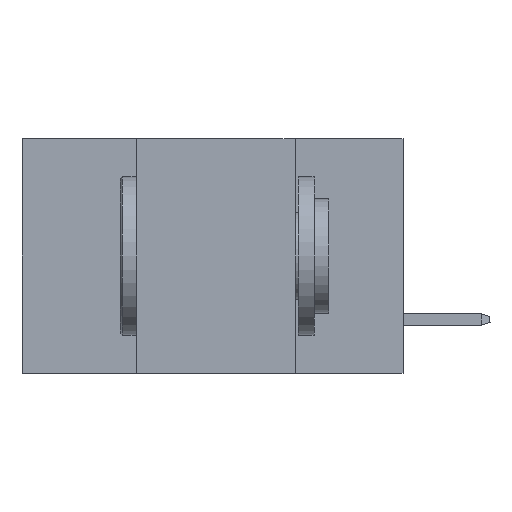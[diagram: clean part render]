
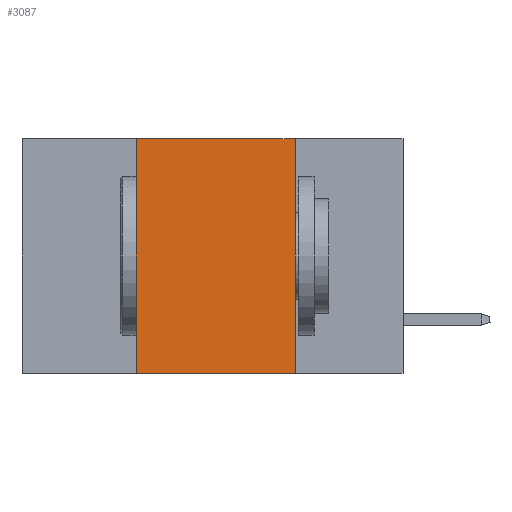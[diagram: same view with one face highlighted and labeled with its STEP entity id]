
A CAD part, left-side view. The second image highlights one B-rep face of the part: STEP entity #3087.
In plain terms, the highlighted planar face has unit normal (-1, 0, 0).
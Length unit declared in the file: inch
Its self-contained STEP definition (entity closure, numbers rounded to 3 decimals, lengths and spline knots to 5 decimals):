
#772 = LINE ( 'NONE', #17700, #2899 ) ;
#1474 = CARTESIAN_POINT ( 'NONE',  ( 0., 0.6, 0. ) ) ;
#1555 = EDGE_CURVE ( 'NONE', #10267, #7672, #14906, .T. ) ;
#1902 = VECTOR ( 'NONE', #2129, 39.37008 ) ;
#2129 = DIRECTION ( 'NONE',  ( 0., -1., 0. ) ) ;
#2788 = FACE_OUTER_BOUND ( 'NONE', #7669, .T. ) ;
#2899 = VECTOR ( 'NONE', #7911, 39.37008 ) ;
#3087 = ADVANCED_FACE ( 'NONE', ( #2788 ), #8455, .F. ) ;
#3581 = VERTEX_POINT ( 'NONE', #17547 ) ;
#4168 = VECTOR ( 'NONE', #13461, 39.37008 ) ;
#5993 = VECTOR ( 'NONE', #18047, 39.37008 ) ;
#6473 = CARTESIAN_POINT ( 'NONE',  ( 0., 0.17, -0.37 ) ) ;
#6506 = CARTESIAN_POINT ( 'NONE',  ( 0., 0.6, -0.37 ) ) ;
#7064 = CARTESIAN_POINT ( 'NONE',  ( 0., 0.6, 0. ) ) ;
#7388 = EDGE_CURVE ( 'NONE', #10267, #12118, #772, .T. ) ;
#7408 = ORIENTED_EDGE ( 'NONE', *, *, #16161, .F. ) ;
#7669 = EDGE_LOOP ( 'NONE', ( #12595, #7408, #10098, #14157 ) ) ;
#7672 = VERTEX_POINT ( 'NONE', #6473 ) ;
#7911 = DIRECTION ( 'NONE',  ( 0., 0., 1. ) ) ;
#8455 = PLANE ( 'NONE',  #10030 ) ;
#9948 = DIRECTION ( 'NONE',  ( 0., 0., -1. ) ) ;
#10030 = AXIS2_PLACEMENT_3D ( 'NONE', #7064, #12706, #9948 ) ;
#10098 = ORIENTED_EDGE ( 'NONE', *, *, #7388, .F. ) ;
#10247 = CARTESIAN_POINT ( 'NONE',  ( 0., 0.42, -0.37 ) ) ;
#10267 = VERTEX_POINT ( 'NONE', #10247 ) ;
#12118 = VERTEX_POINT ( 'NONE', #16963 ) ;
#12227 = EDGE_CURVE ( 'NONE', #3581, #7672, #16307, .T. ) ;
#12595 = ORIENTED_EDGE ( 'NONE', *, *, #12227, .F. ) ;
#12706 = DIRECTION ( 'NONE',  ( 1., 0., 0. ) ) ;
#13461 = DIRECTION ( 'NONE',  ( 0., 0., -1. ) ) ;
#14157 = ORIENTED_EDGE ( 'NONE', *, *, #1555, .T. ) ;
#14165 = LINE ( 'NONE', #1474, #5993 ) ;
#14843 = CARTESIAN_POINT ( 'NONE',  ( 0., 0.17, 0. ) ) ;
#14906 = LINE ( 'NONE', #6506, #1902 ) ;
#16161 = EDGE_CURVE ( 'NONE', #12118, #3581, #14165, .T. ) ;
#16307 = LINE ( 'NONE', #14843, #4168 ) ;
#16963 = CARTESIAN_POINT ( 'NONE',  ( 0., 0.42, 0. ) ) ;
#17547 = CARTESIAN_POINT ( 'NONE',  ( 0., 0.17, 0. ) ) ;
#17700 = CARTESIAN_POINT ( 'NONE',  ( 0., 0.42, 0. ) ) ;
#18047 = DIRECTION ( 'NONE',  ( 0., -1., 0. ) ) ;
